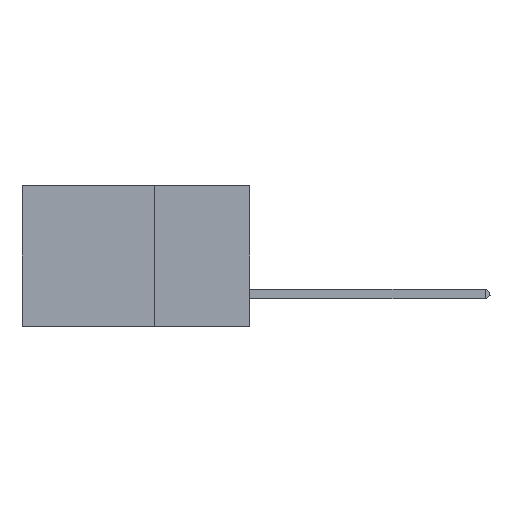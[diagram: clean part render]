
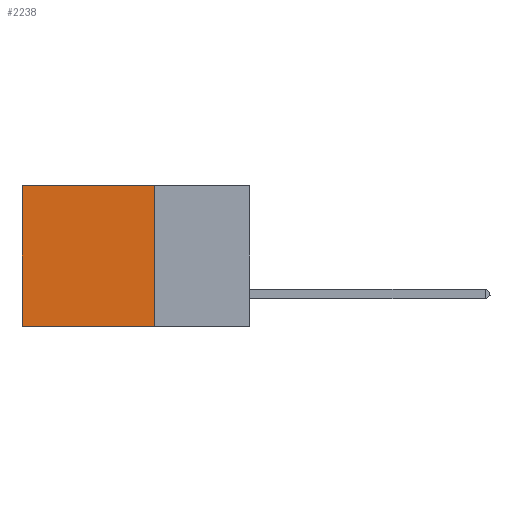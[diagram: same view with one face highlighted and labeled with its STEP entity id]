
A CAD part, left-side view. The second image highlights one B-rep face of the part: STEP entity #2238.
In plain terms, the highlighted planar face has unit normal (-1, 0, 0).
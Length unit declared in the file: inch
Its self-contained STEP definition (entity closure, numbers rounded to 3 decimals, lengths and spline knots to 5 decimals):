
#753 = PLANE ( 'NONE',  #1608 ) ;
#867 = EDGE_CURVE ( 'NONE', #5096, #3961, #15938, .T. ) ;
#1144 = VECTOR ( 'NONE', #14304, 39.37008 ) ;
#1264 = LINE ( 'NONE', #15968, #16617 ) ;
#1440 = ORIENTED_EDGE ( 'NONE', *, *, #16406, .T. ) ;
#1465 = EDGE_LOOP ( 'NONE', ( #14497, #9261, #10358, #1440 ) ) ;
#1608 = AXIS2_PLACEMENT_3D ( 'NONE', #15922, #11745, #17275 ) ;
#1768 = VECTOR ( 'NONE', #5283, 39.37008 ) ;
#1796 = CARTESIAN_POINT ( 'NONE',  ( 0.2875, 0.25, -0.37 ) ) ;
#2238 = ADVANCED_FACE ( 'NONE', ( #17367 ), #753, .F. ) ;
#3067 = VERTEX_POINT ( 'NONE', #7491 ) ;
#3462 = LINE ( 'NONE', #8583, #9921 ) ;
#3644 = EDGE_CURVE ( 'NONE', #3067, #5096, #3462, .T. ) ;
#3961 = VERTEX_POINT ( 'NONE', #9462 ) ;
#3991 = VERTEX_POINT ( 'NONE', #8203 ) ;
#5096 = VERTEX_POINT ( 'NONE', #11675 ) ;
#5283 = DIRECTION ( 'NONE',  ( 0., 1., 0. ) ) ;
#6052 = EDGE_CURVE ( 'NONE', #3991, #3961, #1264, .T. ) ;
#7491 = CARTESIAN_POINT ( 'NONE',  ( 0.2875, 0.25, 0. ) ) ;
#7971 = CARTESIAN_POINT ( 'NONE',  ( 0.2875, 0.25, 0. ) ) ;
#8203 = CARTESIAN_POINT ( 'NONE',  ( 0.2875, 0.6, 0. ) ) ;
#8583 = CARTESIAN_POINT ( 'NONE',  ( 0.2875, 0.25, 0. ) ) ;
#8677 = DIRECTION ( 'NONE',  ( 0., 0., -1. ) ) ;
#9261 = ORIENTED_EDGE ( 'NONE', *, *, #867, .F. ) ;
#9355 = DIRECTION ( 'NONE',  ( 0., 0., -1. ) ) ;
#9462 = CARTESIAN_POINT ( 'NONE',  ( 0.2875, 0.6, -0.37 ) ) ;
#9921 = VECTOR ( 'NONE', #8677, 39.37008 ) ;
#10358 = ORIENTED_EDGE ( 'NONE', *, *, #3644, .F. ) ;
#10580 = LINE ( 'NONE', #7971, #1768 ) ;
#11675 = CARTESIAN_POINT ( 'NONE',  ( 0.2875, 0.25, -0.37 ) ) ;
#11745 = DIRECTION ( 'NONE',  ( 1., 0., 0. ) ) ;
#14304 = DIRECTION ( 'NONE',  ( 0., 1., 0. ) ) ;
#14497 = ORIENTED_EDGE ( 'NONE', *, *, #6052, .T. ) ;
#15922 = CARTESIAN_POINT ( 'NONE',  ( 0.2875, 0.25, 0. ) ) ;
#15938 = LINE ( 'NONE', #1796, #1144 ) ;
#15968 = CARTESIAN_POINT ( 'NONE',  ( 0.2875, 0.6, 0. ) ) ;
#16406 = EDGE_CURVE ( 'NONE', #3067, #3991, #10580, .T. ) ;
#16617 = VECTOR ( 'NONE', #9355, 39.37008 ) ;
#17275 = DIRECTION ( 'NONE',  ( 0., 0., -1. ) ) ;
#17367 = FACE_OUTER_BOUND ( 'NONE', #1465, .T. ) ;
